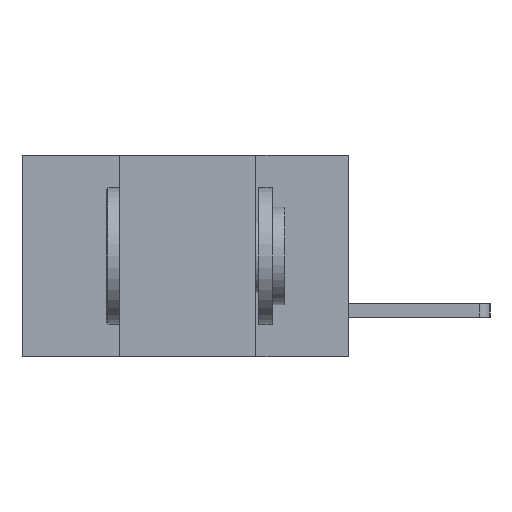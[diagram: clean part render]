
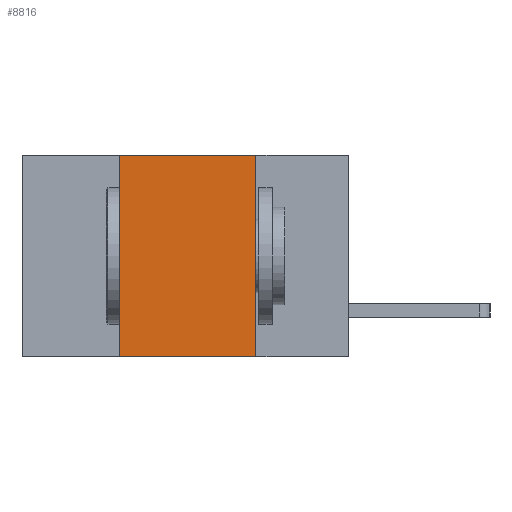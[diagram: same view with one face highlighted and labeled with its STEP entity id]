
A CAD part, left-side view. The second image highlights one B-rep face of the part: STEP entity #8816.
In plain terms, the highlighted planar face has unit normal (-1, 0, 0).
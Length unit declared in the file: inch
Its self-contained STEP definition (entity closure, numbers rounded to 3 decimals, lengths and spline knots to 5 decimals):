
#661 = LINE ( 'NONE', #3220, #2912 ) ;
#871 = LINE ( 'NONE', #4957, #5039 ) ;
#1122 = VERTEX_POINT ( 'NONE', #10447 ) ;
#1234 = CARTESIAN_POINT ( 'NONE',  ( 0., 0.6, -0.37 ) ) ;
#1503 = EDGE_LOOP ( 'NONE', ( #3621, #10196, #6139, #8578 ) ) ;
#2183 = FACE_OUTER_BOUND ( 'NONE', #1503, .T. ) ;
#2385 = EDGE_CURVE ( 'NONE', #6243, #6708, #871, .T. ) ;
#2912 = VECTOR ( 'NONE', #8016, 39.37008 ) ;
#3220 = CARTESIAN_POINT ( 'NONE',  ( 0., 0.17, 0. ) ) ;
#3268 = VERTEX_POINT ( 'NONE', #6478 ) ;
#3588 = EDGE_CURVE ( 'NONE', #6708, #3268, #10399, .T. ) ;
#3621 = ORIENTED_EDGE ( 'NONE', *, *, #4767, .F. ) ;
#4767 = EDGE_CURVE ( 'NONE', #3268, #1122, #661, .T. ) ;
#4792 = DIRECTION ( 'NONE',  ( 1., 0., 0. ) ) ;
#4832 = AXIS2_PLACEMENT_3D ( 'NONE', #8735, #4792, #10299 ) ;
#4957 = CARTESIAN_POINT ( 'NONE',  ( 0., 0.42, 0. ) ) ;
#5039 = VECTOR ( 'NONE', #7048, 39.37008 ) ;
#5579 = CARTESIAN_POINT ( 'NONE',  ( 0., 0.6, 0. ) ) ;
#6139 = ORIENTED_EDGE ( 'NONE', *, *, #2385, .F. ) ;
#6243 = VERTEX_POINT ( 'NONE', #7678 ) ;
#6478 = CARTESIAN_POINT ( 'NONE',  ( 0., 0.17, 0. ) ) ;
#6661 = CARTESIAN_POINT ( 'NONE',  ( 0., 0.42, 0. ) ) ;
#6708 = VERTEX_POINT ( 'NONE', #6661 ) ;
#7048 = DIRECTION ( 'NONE',  ( 0., 0., 1. ) ) ;
#7173 = PLANE ( 'NONE',  #4832 ) ;
#7678 = CARTESIAN_POINT ( 'NONE',  ( 0., 0.42, -0.37 ) ) ;
#7782 = DIRECTION ( 'NONE',  ( 0., -1., 0. ) ) ;
#7825 = VECTOR ( 'NONE', #7782, 39.37008 ) ;
#8016 = DIRECTION ( 'NONE',  ( 0., 0., -1. ) ) ;
#8578 = ORIENTED_EDGE ( 'NONE', *, *, #9267, .T. ) ;
#8735 = CARTESIAN_POINT ( 'NONE',  ( 0., 0.6, 0. ) ) ;
#8816 = ADVANCED_FACE ( 'NONE', ( #2183 ), #7173, .F. ) ;
#9267 = EDGE_CURVE ( 'NONE', #6243, #1122, #10139, .T. ) ;
#10081 = DIRECTION ( 'NONE',  ( 0., -1., 0. ) ) ;
#10139 = LINE ( 'NONE', #1234, #7825 ) ;
#10148 = VECTOR ( 'NONE', #10081, 39.37008 ) ;
#10196 = ORIENTED_EDGE ( 'NONE', *, *, #3588, .F. ) ;
#10299 = DIRECTION ( 'NONE',  ( 0., 0., -1. ) ) ;
#10399 = LINE ( 'NONE', #5579, #10148 ) ;
#10447 = CARTESIAN_POINT ( 'NONE',  ( 0., 0.17, -0.37 ) ) ;
